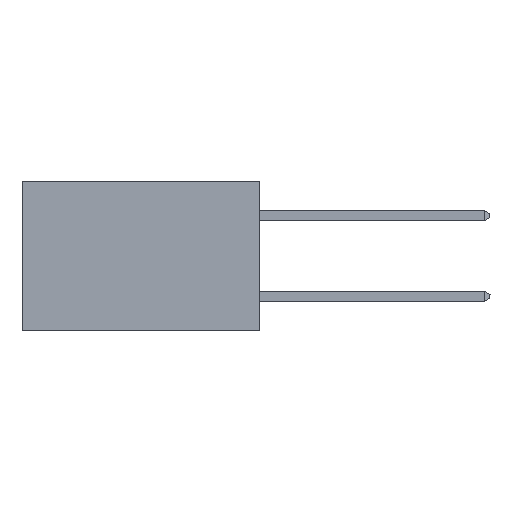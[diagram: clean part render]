
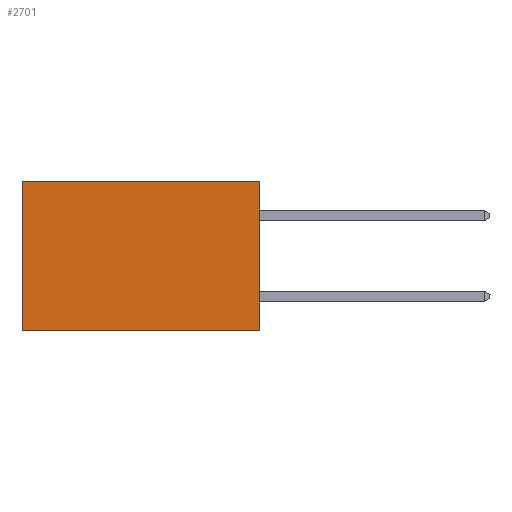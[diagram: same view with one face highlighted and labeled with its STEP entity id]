
A CAD part, left-side view. The second image highlights one B-rep face of the part: STEP entity #2701.
In plain terms, the highlighted planar face has unit normal (-1, 0, 0).
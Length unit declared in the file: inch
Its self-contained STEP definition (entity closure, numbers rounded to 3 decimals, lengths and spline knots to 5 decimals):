
#400 = AXIS2_PLACEMENT_3D ( 'NONE', #1106, #12737, #17687 ) ;
#1106 = CARTESIAN_POINT ( 'NONE',  ( 0.277, 0., -0.37 ) ) ;
#1619 = ORIENTED_EDGE ( 'NONE', *, *, #2246, .F. ) ;
#1808 = EDGE_CURVE ( 'NONE', #18339, #17789, #20201, .T. ) ;
#1975 = VECTOR ( 'NONE', #20147, 39.37008 ) ;
#2246 = EDGE_CURVE ( 'NONE', #4809, #10537, #15295, .T. ) ;
#2701 = ADVANCED_FACE ( 'NONE', ( #19668 ), #4543, .F. ) ;
#4543 = PLANE ( 'NONE',  #400 ) ;
#4809 = VERTEX_POINT ( 'NONE', #19178 ) ;
#5904 = ORIENTED_EDGE ( 'NONE', *, *, #10444, .F. ) ;
#8247 = CARTESIAN_POINT ( 'NONE',  ( 0.277, 0.59, -0.37 ) ) ;
#10444 = EDGE_CURVE ( 'NONE', #18339, #4809, #20078, .T. ) ;
#10537 = VERTEX_POINT ( 'NONE', #20481 ) ;
#10926 = VECTOR ( 'NONE', #14035, 39.37008 ) ;
#11502 = EDGE_LOOP ( 'NONE', ( #14295, #1619, #5904, #20840 ) ) ;
#12205 = CARTESIAN_POINT ( 'NONE',  ( 0.277, 0.59, 0. ) ) ;
#12737 = DIRECTION ( 'NONE',  ( 1., 0., 0. ) ) ;
#13012 = VECTOR ( 'NONE', #18193, 39.37008 ) ;
#13262 = EDGE_CURVE ( 'NONE', #17789, #10537, #13512, .T. ) ;
#13512 = LINE ( 'NONE', #8247, #13012 ) ;
#14035 = DIRECTION ( 'NONE',  ( 0., 1., 0. ) ) ;
#14295 = ORIENTED_EDGE ( 'NONE', *, *, #13262, .T. ) ;
#14484 = CARTESIAN_POINT ( 'NONE',  ( 0.277, 0., 0. ) ) ;
#15295 = LINE ( 'NONE', #20036, #1975 ) ;
#15519 = DIRECTION ( 'NONE',  ( 0., 0., -1. ) ) ;
#16859 = CARTESIAN_POINT ( 'NONE',  ( 0.277, 0., 0. ) ) ;
#17179 = CARTESIAN_POINT ( 'NONE',  ( 0.277, 0., -0.37 ) ) ;
#17687 = DIRECTION ( 'NONE',  ( 0., 0., -1. ) ) ;
#17789 = VERTEX_POINT ( 'NONE', #12205 ) ;
#18193 = DIRECTION ( 'NONE',  ( 0., 0., -1. ) ) ;
#18339 = VERTEX_POINT ( 'NONE', #16859 ) ;
#19178 = CARTESIAN_POINT ( 'NONE',  ( 0.277, 0., -0.37 ) ) ;
#19584 = VECTOR ( 'NONE', #15519, 39.37008 ) ;
#19668 = FACE_OUTER_BOUND ( 'NONE', #11502, .T. ) ;
#20036 = CARTESIAN_POINT ( 'NONE',  ( 0.277, 0., -0.37 ) ) ;
#20078 = LINE ( 'NONE', #17179, #19584 ) ;
#20147 = DIRECTION ( 'NONE',  ( 0., 1., 0. ) ) ;
#20201 = LINE ( 'NONE', #14484, #10926 ) ;
#20481 = CARTESIAN_POINT ( 'NONE',  ( 0.277, 0.59, -0.37 ) ) ;
#20840 = ORIENTED_EDGE ( 'NONE', *, *, #1808, .T. ) ;
